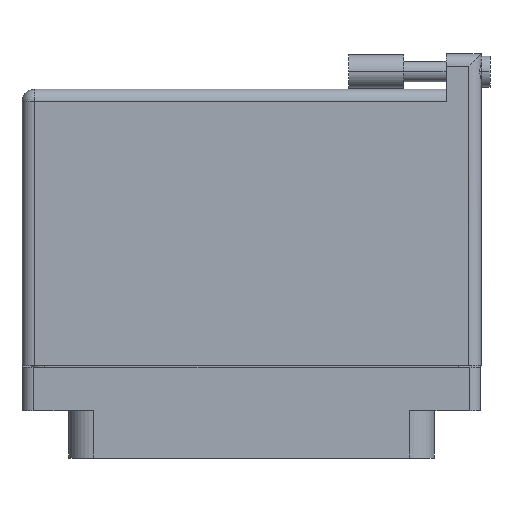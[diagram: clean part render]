
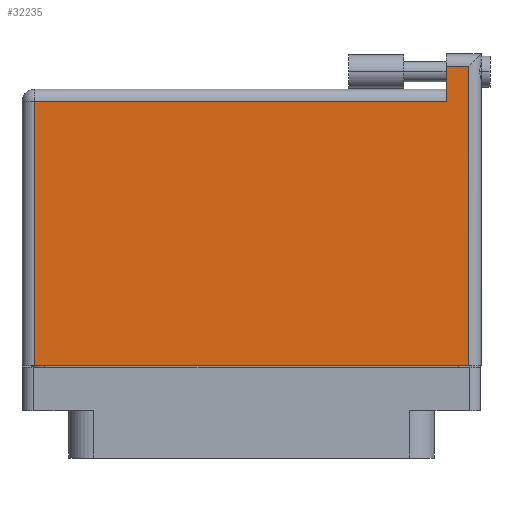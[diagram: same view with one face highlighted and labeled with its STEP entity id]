
A CAD part, front view. The second image highlights one B-rep face of the part: STEP entity #32235.
In plain terms, the highlighted face is planar.
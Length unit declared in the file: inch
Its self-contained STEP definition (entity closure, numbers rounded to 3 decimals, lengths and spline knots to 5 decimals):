
#114 = ORIENTED_EDGE ( 'NONE', *, *, #21241, .T. ) ;
#329 = LINE ( 'NONE', #26434, #20259 ) ;
#1872 = VERTEX_POINT ( 'NONE', #27939 ) ;
#2656 = VECTOR ( 'NONE', #16518, 39.37008 ) ;
#2847 = EDGE_CURVE ( 'NONE', #31765, #1872, #16047, .T. ) ;
#4813 = CARTESIAN_POINT ( 'NONE',  ( 1.23, 1.596, 0.4495 ) ) ;
#5512 = DIRECTION ( 'NONE',  ( -1., 0., 0. ) ) ;
#5588 = ORIENTED_EDGE ( 'NONE', *, *, #43253, .T. ) ;
#7966 = CARTESIAN_POINT ( 'NONE',  ( -1.3, 1.396, 0.4495 ) ) ;
#8438 = PLANE ( 'NONE',  #46297 ) ;
#10686 = VERTEX_POINT ( 'NONE', #15605 ) ;
#11037 = VECTOR ( 'NONE', #12758, 39.37008 ) ;
#11086 = ORIENTED_EDGE ( 'NONE', *, *, #48125, .T. ) ;
#11580 = CARTESIAN_POINT ( 'NONE',  ( 1.103, 1.396, 0.4495 ) ) ;
#12758 = DIRECTION ( 'NONE',  ( -1., 0., 0. ) ) ;
#12950 = CARTESIAN_POINT ( 'NONE',  ( 1.23, -0.1, 0.4495 ) ) ;
#13415 = VECTOR ( 'NONE', #14585, 39.37008 ) ;
#14585 = DIRECTION ( 'NONE',  ( 1., 0., 0. ) ) ;
#14649 = VERTEX_POINT ( 'NONE', #12950 ) ;
#15605 = CARTESIAN_POINT ( 'NONE',  ( -1.23, 1.396, 0.4495 ) ) ;
#16047 = LINE ( 'NONE', #16431, #11037 ) ;
#16431 = CARTESIAN_POINT ( 'NONE',  ( -1.3, 1.596, 0.4495 ) ) ;
#16518 = DIRECTION ( 'NONE',  ( 0., -1., 0. ) ) ;
#16867 = CARTESIAN_POINT ( 'NONE',  ( 1.103, 1.666, 0.4495 ) ) ;
#17336 = DIRECTION ( 'NONE',  ( 0., 0., -1. ) ) ;
#18406 = DIRECTION ( 'NONE',  ( 0., -1., 0. ) ) ;
#20259 = VECTOR ( 'NONE', #34313, 39.37008 ) ;
#21235 = EDGE_CURVE ( 'NONE', #14649, #31765, #329, .T. ) ;
#21241 = EDGE_CURVE ( 'NONE', #25837, #14649, #34652, .T. ) ;
#22751 = CARTESIAN_POINT ( 'NONE',  ( -1.23, -0.1, 0.4495 ) ) ;
#22905 = ORIENTED_EDGE ( 'NONE', *, *, #2847, .T. ) ;
#25837 = VERTEX_POINT ( 'NONE', #44722 ) ;
#26434 = CARTESIAN_POINT ( 'NONE',  ( 1.23, 1.666, 0.4495 ) ) ;
#26987 = VECTOR ( 'NONE', #18406, 39.37008 ) ;
#27939 = CARTESIAN_POINT ( 'NONE',  ( 1.103, 1.596, 0.4495 ) ) ;
#28583 = ORIENTED_EDGE ( 'NONE', *, *, #21235, .T. ) ;
#30395 = ORIENTED_EDGE ( 'NONE', *, *, #36723, .T. ) ;
#31765 = VERTEX_POINT ( 'NONE', #4813 ) ;
#32235 = ADVANCED_FACE ( 'NONE', ( #34470 ), #8438, .F. ) ;
#34313 = DIRECTION ( 'NONE',  ( 0., 1., 0. ) ) ;
#34470 = FACE_OUTER_BOUND ( 'NONE', #40302, .T. ) ;
#34485 = CARTESIAN_POINT ( 'NONE',  ( -1.3, -0.1, 0.4495 ) ) ;
#34652 = LINE ( 'NONE', #34485, #13415 ) ;
#36351 = CARTESIAN_POINT ( 'NONE',  ( -1.3, 1.466, 0.4495 ) ) ;
#36723 = EDGE_CURVE ( 'NONE', #1872, #46714, #43909, .T. ) ;
#37021 = LINE ( 'NONE', #22751, #26987 ) ;
#39940 = DIRECTION ( 'NONE',  ( -1., 0., 0. ) ) ;
#40302 = EDGE_LOOP ( 'NONE', ( #114, #28583, #22905, #30395, #5588, #11086 ) ) ;
#42481 = VECTOR ( 'NONE', #39940, 39.37008 ) ;
#43253 = EDGE_CURVE ( 'NONE', #46714, #10686, #51192, .T. ) ;
#43909 = LINE ( 'NONE', #16867, #2656 ) ;
#44722 = CARTESIAN_POINT ( 'NONE',  ( -1.23, -0.1, 0.4495 ) ) ;
#46297 = AXIS2_PLACEMENT_3D ( 'NONE', #36351, #17336, #5512 ) ;
#46714 = VERTEX_POINT ( 'NONE', #11580 ) ;
#48125 = EDGE_CURVE ( 'NONE', #10686, #25837, #37021, .T. ) ;
#51192 = LINE ( 'NONE', #7966, #42481 ) ;
